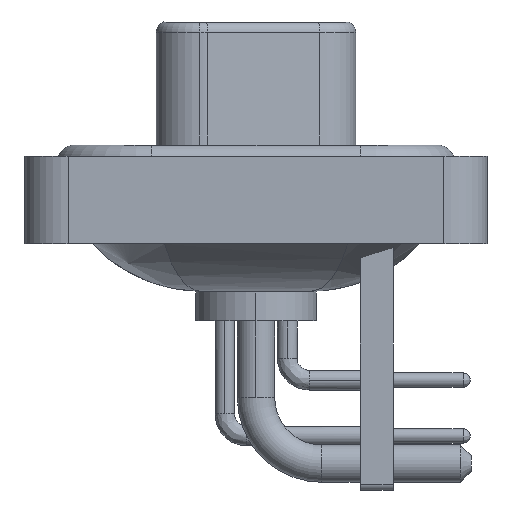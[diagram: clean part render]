
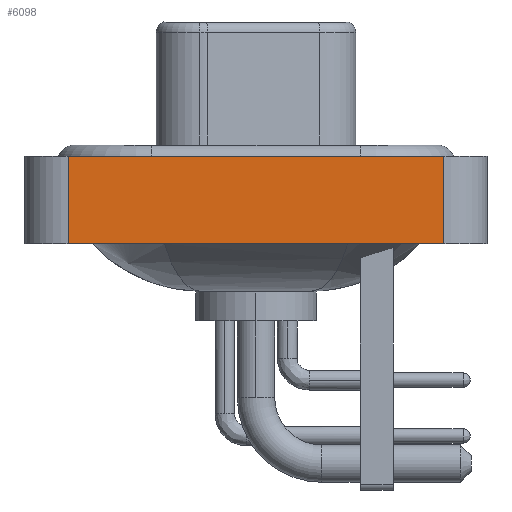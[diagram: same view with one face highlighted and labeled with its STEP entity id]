
A CAD part, left-side view. The second image highlights one B-rep face of the part: STEP entity #6098.
In plain terms, the highlighted planar face has unit normal (-1, 0, 0).
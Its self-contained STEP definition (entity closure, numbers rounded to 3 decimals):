
#678 = LINE ( 'NONE', #4903, #8520 ) ;
#937 = DIRECTION ( 'NONE',  ( 0., 0., 1. ) ) ;
#1008 = VERTEX_POINT ( 'NONE', #19241 ) ;
#2531 = ORIENTED_EDGE ( 'NONE', *, *, #21829, .F. ) ;
#2540 = CARTESIAN_POINT ( 'NONE',  ( -7.3, -8.55, -3.6 ) ) ;
#2945 = ORIENTED_EDGE ( 'NONE', *, *, #6181, .T. ) ;
#4451 = AXIS2_PLACEMENT_3D ( 'NONE', #16162, #23969, #5032 ) ;
#4779 = CARTESIAN_POINT ( 'NONE',  ( -7.3, 8.55, -3.6 ) ) ;
#4903 = CARTESIAN_POINT ( 'NONE',  ( -7.3, -8.55, -3.6 ) ) ;
#5032 = DIRECTION ( 'NONE',  ( 0., 0., 1. ) ) ;
#6098 = ADVANCED_FACE ( 'NONE', ( #16549 ), #6824, .T. ) ;
#6181 = EDGE_CURVE ( 'NONE', #6370, #23046, #678, .T. ) ;
#6370 = VERTEX_POINT ( 'NONE', #2540 ) ;
#6388 = CARTESIAN_POINT ( 'NONE',  ( -7.3, -8.55, 0.4 ) ) ;
#6760 = CARTESIAN_POINT ( 'NONE',  ( -7.3, -8.55, -3.6 ) ) ;
#6824 = PLANE ( 'NONE',  #4451 ) ;
#7177 = VERTEX_POINT ( 'NONE', #13359 ) ;
#8520 = VECTOR ( 'NONE', #937, 1000. ) ;
#9270 = EDGE_CURVE ( 'NONE', #7177, #6370, #16490, .T. ) ;
#10376 = LINE ( 'NONE', #4779, #12337 ) ;
#10442 = DIRECTION ( 'NONE',  ( 0., -1., 0. ) ) ;
#10503 = DIRECTION ( 'NONE',  ( 0., 0., 1. ) ) ;
#10508 = LINE ( 'NONE', #22449, #12391 ) ;
#10854 = VECTOR ( 'NONE', #10442, 1000. ) ;
#12337 = VECTOR ( 'NONE', #10503, 1000. ) ;
#12391 = VECTOR ( 'NONE', #18344, 1000. ) ;
#13359 = CARTESIAN_POINT ( 'NONE',  ( -7.3, 8.55, -3.6 ) ) ;
#13968 = ORIENTED_EDGE ( 'NONE', *, *, #17169, .F. ) ;
#14818 = EDGE_LOOP ( 'NONE', ( #2945, #2531, #13968, #18543 ) ) ;
#16162 = CARTESIAN_POINT ( 'NONE',  ( -7.3, -8.55, -3.6 ) ) ;
#16490 = LINE ( 'NONE', #6760, #10854 ) ;
#16549 = FACE_OUTER_BOUND ( 'NONE', #14818, .T. ) ;
#17169 = EDGE_CURVE ( 'NONE', #7177, #1008, #10376, .T. ) ;
#18344 = DIRECTION ( 'NONE',  ( 0., -1., 0. ) ) ;
#18543 = ORIENTED_EDGE ( 'NONE', *, *, #9270, .T. ) ;
#19241 = CARTESIAN_POINT ( 'NONE',  ( -7.3, 8.55, 0.4 ) ) ;
#21829 = EDGE_CURVE ( 'NONE', #1008, #23046, #10508, .T. ) ;
#22449 = CARTESIAN_POINT ( 'NONE',  ( -7.3, -8.55, 0.4 ) ) ;
#23046 = VERTEX_POINT ( 'NONE', #6388 ) ;
#23969 = DIRECTION ( 'NONE',  ( -1., 0., 0. ) ) ;
